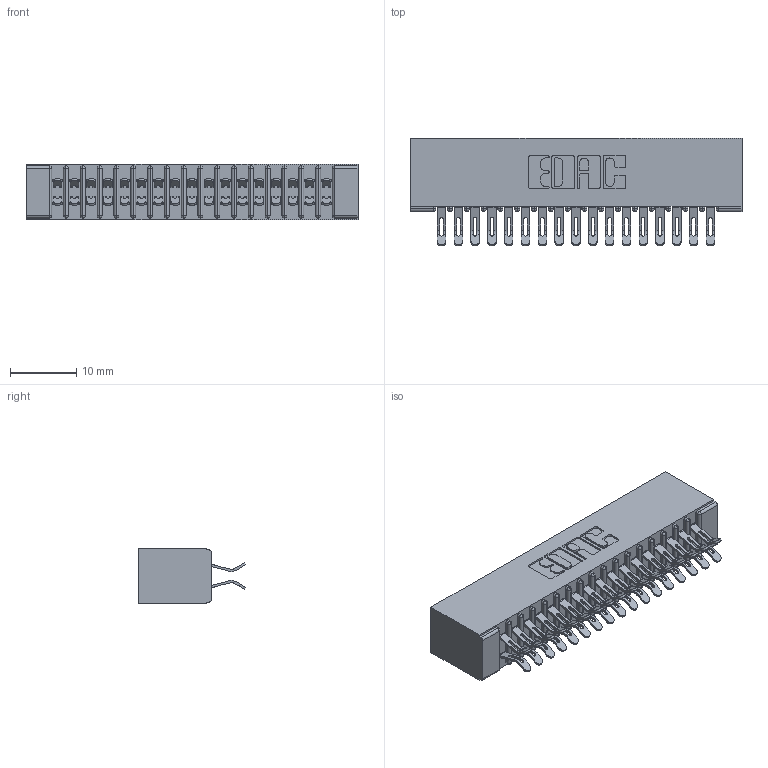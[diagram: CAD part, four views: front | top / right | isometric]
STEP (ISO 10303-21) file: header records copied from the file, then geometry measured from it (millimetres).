
FILE_DESCRIPTION (( 'STEP AP203' ), '1' );
FILE_NAME ('391-034-555-201.STEP', '2018-08-08T22:56:05', ( '' ), ( '' ), 'SwSTEP 2.0', 'SolidWorks 2016', '' );
FILE_SCHEMA (( 'CONFIG_CONTROL_DESIGN' ));
Length unit declared in the file: inch
Products named in the file (3): 341 Part_No Mounting Lugs; 341-292-001_341-292-155; 391-034-555-201
Assembly tree (35 placements, depth 2):
  391-034-555-201
    341 Part_No Mounting Lugs
    341-292-001_341-292-155  x34
Bounding box: 50.16 x 16.31 x 8.38 mm (x, y, z)
Volume: 3041.6 mm3; surface area: 6967.5 mm2
Topology: 35 solids, 35 shells, 2760 faces, 8231 edges, 5358 vertices
Faces by surface type: plane 1492, cylinder 1200, sphere 36, torus 32
Entity records: 24096 total; most frequent: CARTESIAN_POINT 4021, ORIENTED_EDGE 3982, DIRECTION 3909, EDGE_CURVE 1991, LINE 1569, VECTOR 1569, VERTEX_POINT 1266, AXIS2_PLACEMENT_3D 1170
